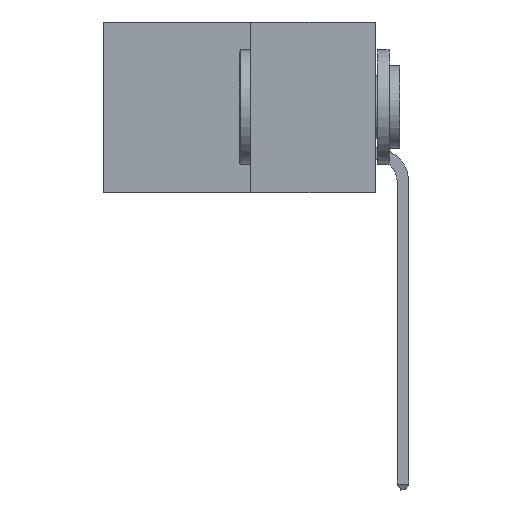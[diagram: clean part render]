
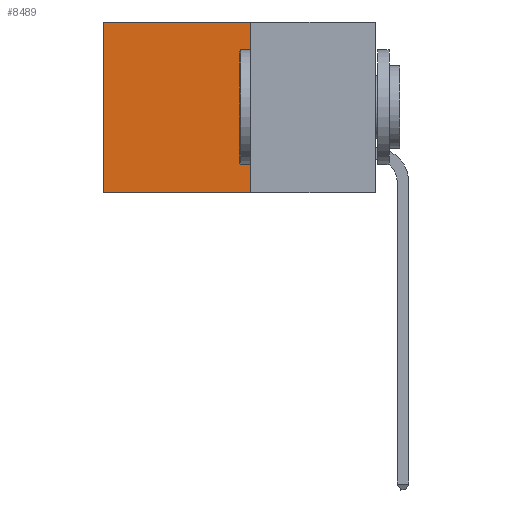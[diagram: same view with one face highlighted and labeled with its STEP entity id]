
A CAD part, left-side view. The second image highlights one B-rep face of the part: STEP entity #8489.
In plain terms, the highlighted planar face has unit normal (-1, 0, 0).
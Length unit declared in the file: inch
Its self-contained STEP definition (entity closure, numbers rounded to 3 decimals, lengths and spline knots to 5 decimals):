
#361 = CARTESIAN_POINT ( 'NONE',  ( 0.277, 0.27, -0.37 ) ) ;
#1410 = LINE ( 'NONE', #13723, #25977 ) ;
#1682 = ORIENTED_EDGE ( 'NONE', *, *, #29659, .F. ) ;
#1908 = DIRECTION ( 'NONE',  ( 0., 0., -1. ) ) ;
#2120 = LINE ( 'NONE', #361, #21031 ) ;
#6466 = LINE ( 'NONE', #31089, #25934 ) ;
#7873 = VERTEX_POINT ( 'NONE', #14336 ) ;
#8489 = ADVANCED_FACE ( 'NONE', ( #20629 ), #21771, .F. ) ;
#9309 = CARTESIAN_POINT ( 'NONE',  ( 0.277, 0.27, 0. ) ) ;
#12037 = CARTESIAN_POINT ( 'NONE',  ( 0.277, 0.27, 0. ) ) ;
#13298 = ORIENTED_EDGE ( 'NONE', *, *, #25912, .F. ) ;
#13723 = CARTESIAN_POINT ( 'NONE',  ( 0.277, 0.27, -0.37 ) ) ;
#14336 = CARTESIAN_POINT ( 'NONE',  ( 0.277, 0.59, 0. ) ) ;
#14999 = CARTESIAN_POINT ( 'NONE',  ( 0.277, 0.59, -0.37 ) ) ;
#16775 = LINE ( 'NONE', #9309, #28849 ) ;
#18203 = ORIENTED_EDGE ( 'NONE', *, *, #26923, .T. ) ;
#19285 = EDGE_CURVE ( 'NONE', #7873, #24034, #6466, .T. ) ;
#19380 = VERTEX_POINT ( 'NONE', #12037 ) ;
#20629 = FACE_OUTER_BOUND ( 'NONE', #29234, .T. ) ;
#21031 = VECTOR ( 'NONE', #29740, 39.37008 ) ;
#21323 = AXIS2_PLACEMENT_3D ( 'NONE', #21430, #21391, #21363 ) ;
#21363 = DIRECTION ( 'NONE',  ( 0., 0., -1. ) ) ;
#21391 = DIRECTION ( 'NONE',  ( 1., 0., 0. ) ) ;
#21430 = CARTESIAN_POINT ( 'NONE',  ( 0.277, 0.27, -0.37 ) ) ;
#21525 = DIRECTION ( 'NONE',  ( 0., 1., 0. ) ) ;
#21771 = PLANE ( 'NONE',  #21323 ) ;
#24034 = VERTEX_POINT ( 'NONE', #14999 ) ;
#25246 = ORIENTED_EDGE ( 'NONE', *, *, #19285, .T. ) ;
#25912 = EDGE_CURVE ( 'NONE', #31099, #24034, #2120, .T. ) ;
#25934 = VECTOR ( 'NONE', #1908, 39.37008 ) ;
#25977 = VECTOR ( 'NONE', #28296, 39.37008 ) ;
#26923 = EDGE_CURVE ( 'NONE', #19380, #7873, #16775, .T. ) ;
#28296 = DIRECTION ( 'NONE',  ( 0., 0., -1. ) ) ;
#28849 = VECTOR ( 'NONE', #21525, 39.37008 ) ;
#29234 = EDGE_LOOP ( 'NONE', ( #25246, #13298, #1682, #18203 ) ) ;
#29659 = EDGE_CURVE ( 'NONE', #19380, #31099, #1410, .T. ) ;
#29740 = DIRECTION ( 'NONE',  ( 0., 1., 0. ) ) ;
#31089 = CARTESIAN_POINT ( 'NONE',  ( 0.277, 0.59, -0.37 ) ) ;
#31099 = VERTEX_POINT ( 'NONE', #31586 ) ;
#31586 = CARTESIAN_POINT ( 'NONE',  ( 0.277, 0.27, -0.37 ) ) ;
